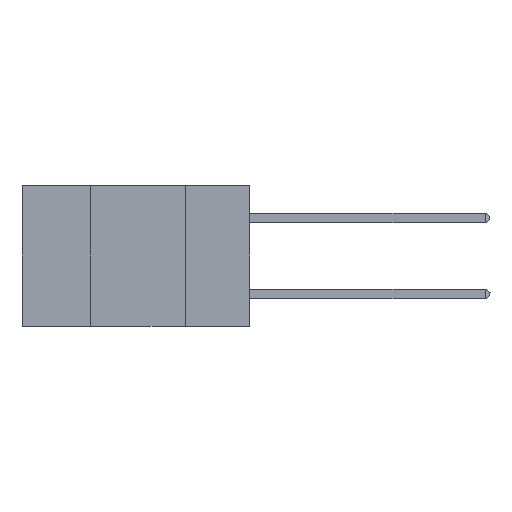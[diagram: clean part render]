
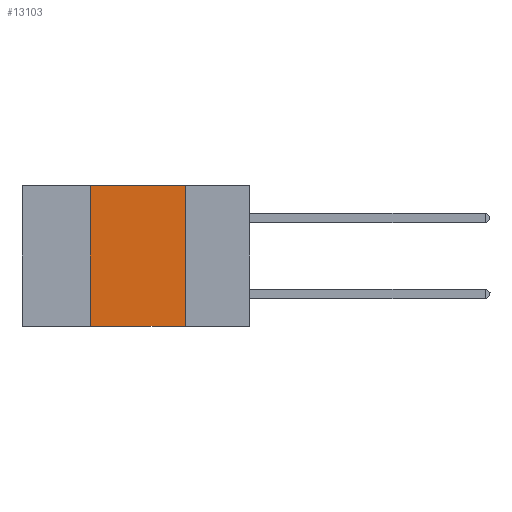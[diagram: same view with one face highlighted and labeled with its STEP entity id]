
A CAD part, left-side view. The second image highlights one B-rep face of the part: STEP entity #13103.
In plain terms, the highlighted planar face has unit normal (-1, 0, 0).
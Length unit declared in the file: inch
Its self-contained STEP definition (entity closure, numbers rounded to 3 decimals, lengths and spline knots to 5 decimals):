
#299 = LINE ( 'NONE', #16768, #12929 ) ;
#1200 = EDGE_CURVE ( 'NONE', #9041, #3923, #299, .T. ) ;
#1448 = ORIENTED_EDGE ( 'NONE', *, *, #10424, .F. ) ;
#1978 = LINE ( 'NONE', #11806, #12588 ) ;
#2594 = EDGE_CURVE ( 'NONE', #9041, #6026, #5151, .T. ) ;
#3485 = VECTOR ( 'NONE', #7492, 39.37008 ) ;
#3923 = VERTEX_POINT ( 'NONE', #7182 ) ;
#4157 = PLANE ( 'NONE',  #11108 ) ;
#4884 = CARTESIAN_POINT ( 'NONE',  ( 0., 0.17, -0.37 ) ) ;
#5151 = LINE ( 'NONE', #6829, #11672 ) ;
#6026 = VERTEX_POINT ( 'NONE', #4884 ) ;
#6259 = CARTESIAN_POINT ( 'NONE',  ( 0., 0.17, 0. ) ) ;
#6639 = ORIENTED_EDGE ( 'NONE', *, *, #16716, .F. ) ;
#6777 = DIRECTION ( 'NONE',  ( 1., 0., 0. ) ) ;
#6829 = CARTESIAN_POINT ( 'NONE',  ( 0., 0.6, -0.37 ) ) ;
#6950 = CARTESIAN_POINT ( 'NONE',  ( 0., 0.6, 0. ) ) ;
#7118 = FACE_OUTER_BOUND ( 'NONE', #7146, .T. ) ;
#7146 = EDGE_LOOP ( 'NONE', ( #6639, #1448, #16359, #11248 ) ) ;
#7182 = CARTESIAN_POINT ( 'NONE',  ( 0., 0.42, 0. ) ) ;
#7492 = DIRECTION ( 'NONE',  ( 0., 0., -1. ) ) ;
#8078 = DIRECTION ( 'NONE',  ( 0., 0., -1. ) ) ;
#8135 = DIRECTION ( 'NONE',  ( 0., -1., 0. ) ) ;
#9041 = VERTEX_POINT ( 'NONE', #13239 ) ;
#10409 = LINE ( 'NONE', #6259, #3485 ) ;
#10424 = EDGE_CURVE ( 'NONE', #3923, #15856, #1978, .T. ) ;
#11108 = AXIS2_PLACEMENT_3D ( 'NONE', #6950, #6777, #8078 ) ;
#11248 = ORIENTED_EDGE ( 'NONE', *, *, #2594, .T. ) ;
#11672 = VECTOR ( 'NONE', #8135, 39.37008 ) ;
#11806 = CARTESIAN_POINT ( 'NONE',  ( 0., 0.6, 0. ) ) ;
#11859 = CARTESIAN_POINT ( 'NONE',  ( 0., 0.17, 0. ) ) ;
#12588 = VECTOR ( 'NONE', #14341, 39.37008 ) ;
#12929 = VECTOR ( 'NONE', #14190, 39.37008 ) ;
#13103 = ADVANCED_FACE ( 'NONE', ( #7118 ), #4157, .F. ) ;
#13239 = CARTESIAN_POINT ( 'NONE',  ( 0., 0.42, -0.37 ) ) ;
#14190 = DIRECTION ( 'NONE',  ( 0., 0., 1. ) ) ;
#14341 = DIRECTION ( 'NONE',  ( 0., -1., 0. ) ) ;
#15856 = VERTEX_POINT ( 'NONE', #11859 ) ;
#16359 = ORIENTED_EDGE ( 'NONE', *, *, #1200, .F. ) ;
#16716 = EDGE_CURVE ( 'NONE', #15856, #6026, #10409, .T. ) ;
#16768 = CARTESIAN_POINT ( 'NONE',  ( 0., 0.42, 0. ) ) ;
